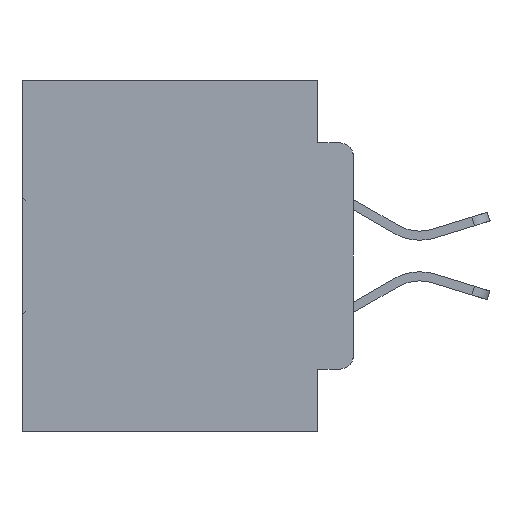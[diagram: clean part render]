
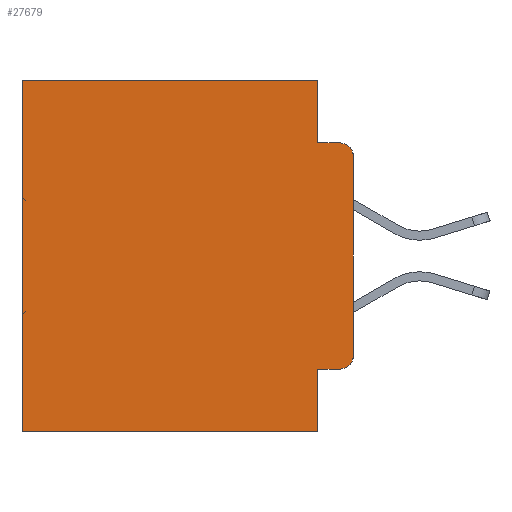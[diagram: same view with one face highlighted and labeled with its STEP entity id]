
A CAD part, left-side view. The second image highlights one B-rep face of the part: STEP entity #27679.
In plain terms, the highlighted planar face has unit normal (-1, 0, 0).
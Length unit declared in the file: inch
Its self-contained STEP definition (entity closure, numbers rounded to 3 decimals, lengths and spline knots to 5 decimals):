
#569 = CARTESIAN_POINT ( 'NONE',  ( 0.298, 0.051, 0. ) ) ;
#1068 = ORIENTED_EDGE ( 'NONE', *, *, #33179, .T. ) ;
#1145 = DIRECTION ( 'NONE',  ( 1., 0., 0. ) ) ;
#2163 = LINE ( 'NONE', #22282, #9840 ) ;
#2214 = EDGE_CURVE ( 'NONE', #5580, #24613, #24593, .T. ) ;
#2664 = LINE ( 'NONE', #4318, #21177 ) ;
#3873 = VERTEX_POINT ( 'NONE', #29011 ) ;
#4119 = CARTESIAN_POINT ( 'NONE',  ( 0.298, 0.02, -0.3915 ) ) ;
#4297 = CARTESIAN_POINT ( 'NONE',  ( 0.298, 0.473, -0.5 ) ) ;
#4318 = CARTESIAN_POINT ( 'NONE',  ( 0.298, 0.051, 0. ) ) ;
#4601 = LINE ( 'NONE', #27087, #21891 ) ;
#5397 = VECTOR ( 'NONE', #5646, 39.37008 ) ;
#5580 = VERTEX_POINT ( 'NONE', #24212 ) ;
#5646 = DIRECTION ( 'NONE',  ( 0., 0., -1. ) ) ;
#5763 = CARTESIAN_POINT ( 'NONE',  ( 0.298, 0., 0. ) ) ;
#6856 = ORIENTED_EDGE ( 'NONE', *, *, #7611, .T. ) ;
#7611 = EDGE_CURVE ( 'NONE', #22483, #31377, #4601, .T. ) ;
#8066 = CARTESIAN_POINT ( 'NONE',  ( 0.298, 0., -0.1085 ) ) ;
#8624 = CARTESIAN_POINT ( 'NONE',  ( 0.298, 0., 0. ) ) ;
#8974 = EDGE_CURVE ( 'NONE', #3873, #19971, #26223, .T. ) ;
#9085 = CIRCLE ( 'NONE', #15430, 0.02 ) ;
#9215 = DIRECTION ( 'NONE',  ( 0., 0., -1. ) ) ;
#9318 = DIRECTION ( 'NONE',  ( -1., 0., 0. ) ) ;
#9840 = VECTOR ( 'NONE', #15313, 39.37008 ) ;
#9930 = VERTEX_POINT ( 'NONE', #29592 ) ;
#10033 = LINE ( 'NONE', #16061, #14449 ) ;
#10072 = EDGE_CURVE ( 'NONE', #19971, #24781, #10033, .T. ) ;
#10075 = LINE ( 'NONE', #569, #29775 ) ;
#10547 = CARTESIAN_POINT ( 'NONE',  ( 0.298, 0., 0. ) ) ;
#12544 = VECTOR ( 'NONE', #15717, 39.37008 ) ;
#12662 = EDGE_CURVE ( 'NONE', #9930, #24781, #2163, .T. ) ;
#13039 = ORIENTED_EDGE ( 'NONE', *, *, #8974, .T. ) ;
#13048 = CARTESIAN_POINT ( 'NONE',  ( 0.298, 0.051, -0.4115 ) ) ;
#13236 = DIRECTION ( 'NONE',  ( 0., -1., 0. ) ) ;
#13476 = DIRECTION ( 'NONE',  ( 0., 0., -1. ) ) ;
#13988 = ORIENTED_EDGE ( 'NONE', *, *, #15094, .F. ) ;
#14177 = AXIS2_PLACEMENT_3D ( 'NONE', #29821, #14756, #32523 ) ;
#14449 = VECTOR ( 'NONE', #13476, 39.37008 ) ;
#14756 = DIRECTION ( 'NONE',  ( -1., 0., 0. ) ) ;
#15093 = ORIENTED_EDGE ( 'NONE', *, *, #2214, .F. ) ;
#15094 = EDGE_CURVE ( 'NONE', #22483, #9930, #10075, .T. ) ;
#15313 = DIRECTION ( 'NONE',  ( 0., 1., 0. ) ) ;
#15430 = AXIS2_PLACEMENT_3D ( 'NONE', #4119, #9318, #9215 ) ;
#15678 = VERTEX_POINT ( 'NONE', #24398 ) ;
#15717 = DIRECTION ( 'NONE',  ( 0., 1., 0. ) ) ;
#16061 = CARTESIAN_POINT ( 'NONE',  ( 0.298, 0.473, 0. ) ) ;
#16217 = CARTESIAN_POINT ( 'NONE',  ( 0.298, 0.473, 0. ) ) ;
#17075 = EDGE_CURVE ( 'NONE', #3873, #5580, #2664, .T. ) ;
#17486 = CIRCLE ( 'NONE', #14177, 0.02 ) ;
#17520 = FACE_OUTER_BOUND ( 'NONE', #26054, .T. ) ;
#18566 = DIRECTION ( 'NONE',  ( 0., 0., -1. ) ) ;
#19408 = DIRECTION ( 'NONE',  ( 0., -1., 0. ) ) ;
#19971 = VERTEX_POINT ( 'NONE', #16217 ) ;
#21177 = VECTOR ( 'NONE', #32670, 39.37008 ) ;
#21618 = PLANE ( 'NONE',  #30334 ) ;
#21891 = VECTOR ( 'NONE', #19408, 39.37008 ) ;
#22282 = CARTESIAN_POINT ( 'NONE',  ( 0.298, 0., -0.5 ) ) ;
#22483 = VERTEX_POINT ( 'NONE', #13048 ) ;
#22650 = CARTESIAN_POINT ( 'NONE',  ( 0.298, 0.02, -0.4115 ) ) ;
#22889 = ORIENTED_EDGE ( 'NONE', *, *, #28148, .T. ) ;
#24212 = CARTESIAN_POINT ( 'NONE',  ( 0.298, 0.051, -0.0885 ) ) ;
#24303 = ORIENTED_EDGE ( 'NONE', *, *, #12662, .F. ) ;
#24398 = CARTESIAN_POINT ( 'NONE',  ( 0.298, 0., -0.3915 ) ) ;
#24593 = LINE ( 'NONE', #26045, #32646 ) ;
#24613 = VERTEX_POINT ( 'NONE', #32109 ) ;
#24781 = VERTEX_POINT ( 'NONE', #4297 ) ;
#24880 = ORIENTED_EDGE ( 'NONE', *, *, #10072, .T. ) ;
#25934 = LINE ( 'NONE', #5763, #5397 ) ;
#26045 = CARTESIAN_POINT ( 'NONE',  ( 0.298, 0.051, -0.0885 ) ) ;
#26054 = EDGE_LOOP ( 'NONE', ( #32489, #22889, #15093, #31269, #13039, #24880, #24303, #13988, #6856, #1068 ) ) ;
#26223 = LINE ( 'NONE', #10547, #12544 ) ;
#26609 = DIRECTION ( 'NONE',  ( 0., 0., -1. ) ) ;
#27087 = CARTESIAN_POINT ( 'NONE',  ( 0.298, 0.051, -0.4115 ) ) ;
#27679 = ADVANCED_FACE ( 'NONE', ( #17520 ), #21618, .F. ) ;
#27892 = EDGE_CURVE ( 'NONE', #29609, #15678, #25934, .T. ) ;
#28148 = EDGE_CURVE ( 'NONE', #29609, #24613, #17486, .T. ) ;
#29011 = CARTESIAN_POINT ( 'NONE',  ( 0.298, 0.051, 0. ) ) ;
#29592 = CARTESIAN_POINT ( 'NONE',  ( 0.298, 0.051, -0.5 ) ) ;
#29609 = VERTEX_POINT ( 'NONE', #8066 ) ;
#29775 = VECTOR ( 'NONE', #18566, 39.37008 ) ;
#29821 = CARTESIAN_POINT ( 'NONE',  ( 0.298, 0.02, -0.1085 ) ) ;
#30334 = AXIS2_PLACEMENT_3D ( 'NONE', #8624, #1145, #26609 ) ;
#31269 = ORIENTED_EDGE ( 'NONE', *, *, #17075, .F. ) ;
#31377 = VERTEX_POINT ( 'NONE', #22650 ) ;
#32109 = CARTESIAN_POINT ( 'NONE',  ( 0.298, 0.02, -0.0885 ) ) ;
#32489 = ORIENTED_EDGE ( 'NONE', *, *, #27892, .F. ) ;
#32523 = DIRECTION ( 'NONE',  ( 0., 0., -1. ) ) ;
#32646 = VECTOR ( 'NONE', #13236, 39.37008 ) ;
#32670 = DIRECTION ( 'NONE',  ( 0., 0., -1. ) ) ;
#33179 = EDGE_CURVE ( 'NONE', #31377, #15678, #9085, .T. ) ;
